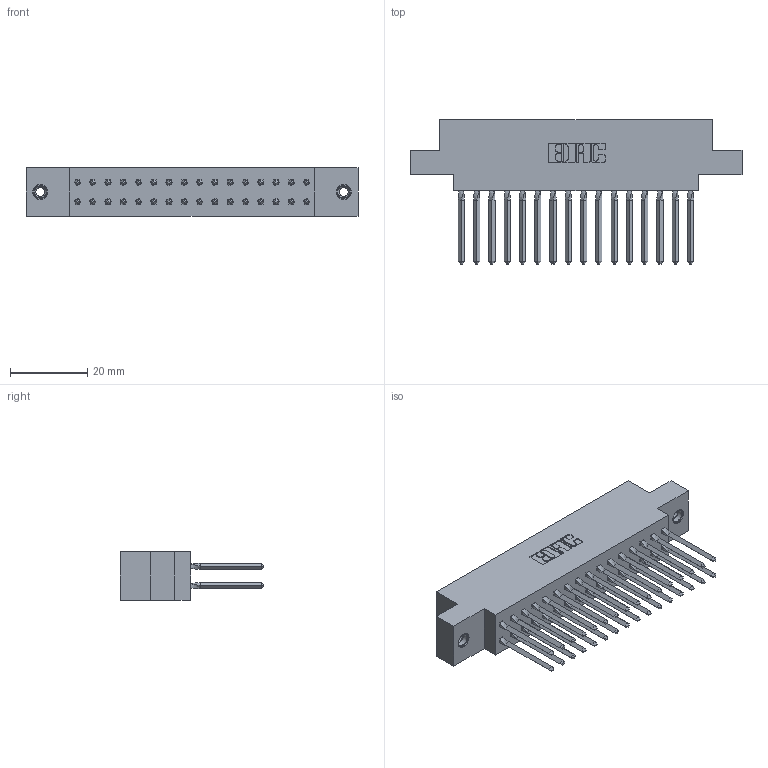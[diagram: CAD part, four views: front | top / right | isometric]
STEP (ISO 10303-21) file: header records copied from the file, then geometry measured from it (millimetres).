
FILE_DESCRIPTION (( 'STEP AP203' ), '1' );
FILE_NAME ('317-032-540-808.STEP', '2020-02-27T21:09:51', ( '' ), ( '' ), 'SwSTEP 2.0', 'SolidWorks 2016', '' );
FILE_SCHEMA (( 'CONFIG_CONTROL_DESIGN' ));
Length unit declared in the file: inch
Products named in the file (4): 317 Part_.156 Dia - TI; 317-290-001_540; 317-032-540-808; 345-250-001_345-250-003-102
Assembly tree (35 placements, depth 2):
  317-032-540-808
    317 Part_.156 Dia - TI
    317-290-001_540  x32
    345-250-001_345-250-003-102  x2
Bounding box: 86.11 x 37.34 x 12.7 mm (x, y, z)
Volume: 13565.7 mm3; surface area: 19265.3 mm2
Topology: 35 solids, 35 shells, 3010 faces, 8315 edges, 5354 vertices
Faces by surface type: plane 2426, cylinder 440, bspline 128, cone 12, torus 4
Entity records: 27941 total; most frequent: CARTESIAN_POINT 5258, ORIENTED_EDGE 4750, DIRECTION 4007, EDGE_CURVE 2375, VECTOR 2099, LINE 2099, VERTEX_POINT 1573, AXIS2_PLACEMENT_3D 954
